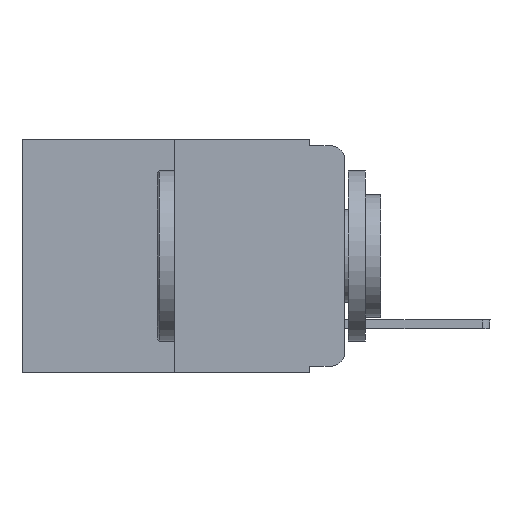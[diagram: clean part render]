
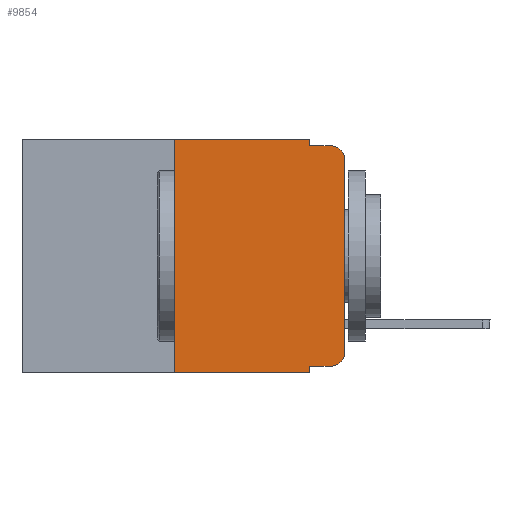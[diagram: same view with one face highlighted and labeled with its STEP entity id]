
A CAD part, left-side view. The second image highlights one B-rep face of the part: STEP entity #9854.
In plain terms, the highlighted planar face has unit normal (-1, 0, 0).
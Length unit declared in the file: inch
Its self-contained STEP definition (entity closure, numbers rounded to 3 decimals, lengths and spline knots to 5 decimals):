
#209 = DIRECTION ( 'NONE',  ( 0., -1., 0. ) ) ;
#552 = VERTEX_POINT ( 'NONE', #6291 ) ;
#686 = VECTOR ( 'NONE', #209, 39.37008 ) ;
#919 = EDGE_CURVE ( 'NONE', #14652, #11674, #9629, .T. ) ;
#1417 = ORIENTED_EDGE ( 'NONE', *, *, #19301, .F. ) ;
#1532 = DIRECTION ( 'NONE',  ( 0., 0., -1. ) ) ;
#1660 = VERTEX_POINT ( 'NONE', #18751 ) ;
#1705 = VERTEX_POINT ( 'NONE', #12756 ) ;
#1905 = EDGE_CURVE ( 'NONE', #5486, #1705, #5115, .T. ) ;
#2225 = EDGE_CURVE ( 'NONE', #14652, #9755, #11635, .T. ) ;
#2271 = ORIENTED_EDGE ( 'NONE', *, *, #5513, .F. ) ;
#2511 = DIRECTION ( 'NONE',  ( -1., 0., 0. ) ) ;
#2537 = CARTESIAN_POINT ( 'NONE',  ( 0., 0.02, -0.01 ) ) ;
#2592 = LINE ( 'NONE', #7316, #13787 ) ;
#2668 = DIRECTION ( 'NONE',  ( -1., 0., 0. ) ) ;
#3148 = EDGE_CURVE ( 'NONE', #552, #21442, #18914, .T. ) ;
#3550 = EDGE_CURVE ( 'NONE', #8674, #1660, #5572, .T. ) ;
#3687 = CARTESIAN_POINT ( 'NONE',  ( 0., 0.051, 0. ) ) ;
#3995 = VECTOR ( 'NONE', #19295, 39.37008 ) ;
#4328 = CARTESIAN_POINT ( 'NONE',  ( 0., 0.25, -0.343 ) ) ;
#5115 = LINE ( 'NONE', #20391, #686 ) ;
#5486 = VERTEX_POINT ( 'NONE', #11490 ) ;
#5513 = EDGE_CURVE ( 'NONE', #10759, #552, #10930, .T. ) ;
#5572 = LINE ( 'NONE', #9108, #3995 ) ;
#5699 = ORIENTED_EDGE ( 'NONE', *, *, #3148, .F. ) ;
#5952 = CARTESIAN_POINT ( 'NONE',  ( 0., 0.051, -0.343 ) ) ;
#6035 = EDGE_CURVE ( 'NONE', #1660, #21442, #16421, .T. ) ;
#6173 = CARTESIAN_POINT ( 'NONE',  ( 0., 0., -0.313 ) ) ;
#6238 = DIRECTION ( 'NONE',  ( 0., 0., -1. ) ) ;
#6291 = CARTESIAN_POINT ( 'NONE',  ( 0., 0.051, -0.01 ) ) ;
#6382 = AXIS2_PLACEMENT_3D ( 'NONE', #12459, #2511, #7522 ) ;
#6492 = CARTESIAN_POINT ( 'NONE',  ( 0., 0.051, 0. ) ) ;
#6511 = VECTOR ( 'NONE', #1532, 39.37008 ) ;
#6634 = ORIENTED_EDGE ( 'NONE', *, *, #18701, .T. ) ;
#7316 = CARTESIAN_POINT ( 'NONE',  ( 0., 0.473, 0. ) ) ;
#7522 = DIRECTION ( 'NONE',  ( 0., 0., -1. ) ) ;
#7699 = CARTESIAN_POINT ( 'NONE',  ( 0., 0.02, -0.03 ) ) ;
#7962 = CARTESIAN_POINT ( 'NONE',  ( 0., 0.25, 0. ) ) ;
#8349 = VECTOR ( 'NONE', #6238, 39.37008 ) ;
#8395 = CIRCLE ( 'NONE', #6382, 0.02 ) ;
#8673 = ORIENTED_EDGE ( 'NONE', *, *, #1905, .T. ) ;
#8674 = VERTEX_POINT ( 'NONE', #6173 ) ;
#9057 = PLANE ( 'NONE',  #16336 ) ;
#9108 = CARTESIAN_POINT ( 'NONE',  ( 0., 0., 0. ) ) ;
#9545 = CARTESIAN_POINT ( 'NONE',  ( 0., 0.051, 0. ) ) ;
#9629 = LINE ( 'NONE', #12203, #13524 ) ;
#9734 = ORIENTED_EDGE ( 'NONE', *, *, #10953, .F. ) ;
#9755 = VERTEX_POINT ( 'NONE', #5952 ) ;
#9854 = ADVANCED_FACE ( 'NONE', ( #20655 ), #9057, .F. ) ;
#9924 = ORIENTED_EDGE ( 'NONE', *, *, #919, .F. ) ;
#10759 = VERTEX_POINT ( 'NONE', #3687 ) ;
#10767 = EDGE_LOOP ( 'NONE', ( #15612, #12100, #5699, #2271, #9734, #9924, #16458, #1417, #8673, #6634 ) ) ;
#10930 = LINE ( 'NONE', #6492, #6511 ) ;
#10953 = EDGE_CURVE ( 'NONE', #11674, #10759, #2592, .T. ) ;
#11490 = CARTESIAN_POINT ( 'NONE',  ( 0., 0.051, -0.333 ) ) ;
#11635 = LINE ( 'NONE', #20192, #20008 ) ;
#11674 = VERTEX_POINT ( 'NONE', #7962 ) ;
#12100 = ORIENTED_EDGE ( 'NONE', *, *, #6035, .T. ) ;
#12203 = CARTESIAN_POINT ( 'NONE',  ( 0., 0.25, 0. ) ) ;
#12459 = CARTESIAN_POINT ( 'NONE',  ( 0., 0.02, -0.313 ) ) ;
#12756 = CARTESIAN_POINT ( 'NONE',  ( 0., 0.02, -0.333 ) ) ;
#12782 = DIRECTION ( 'NONE',  ( 0., 0., -1. ) ) ;
#13524 = VECTOR ( 'NONE', #13876, 39.37008 ) ;
#13584 = LINE ( 'NONE', #9545, #8349 ) ;
#13787 = VECTOR ( 'NONE', #18991, 39.37008 ) ;
#13876 = DIRECTION ( 'NONE',  ( 0., 0., 1. ) ) ;
#13926 = CARTESIAN_POINT ( 'NONE',  ( 0., 0.473, 0. ) ) ;
#14135 = DIRECTION ( 'NONE',  ( 0., 0., -1. ) ) ;
#14652 = VERTEX_POINT ( 'NONE', #4328 ) ;
#15612 = ORIENTED_EDGE ( 'NONE', *, *, #3550, .T. ) ;
#16336 = AXIS2_PLACEMENT_3D ( 'NONE', #13926, #20740, #14135 ) ;
#16421 = CIRCLE ( 'NONE', #19184, 0.02 ) ;
#16458 = ORIENTED_EDGE ( 'NONE', *, *, #2225, .T. ) ;
#16645 = DIRECTION ( 'NONE',  ( 0., -1., 0. ) ) ;
#16929 = DIRECTION ( 'NONE',  ( 0., -1., 0. ) ) ;
#18014 = CARTESIAN_POINT ( 'NONE',  ( 0., 0.051, -0.01 ) ) ;
#18409 = VECTOR ( 'NONE', #16645, 39.37008 ) ;
#18701 = EDGE_CURVE ( 'NONE', #1705, #8674, #8395, .T. ) ;
#18751 = CARTESIAN_POINT ( 'NONE',  ( 0., 0., -0.03 ) ) ;
#18914 = LINE ( 'NONE', #18014, #18409 ) ;
#18991 = DIRECTION ( 'NONE',  ( 0., -1., 0. ) ) ;
#19184 = AXIS2_PLACEMENT_3D ( 'NONE', #7699, #2668, #12782 ) ;
#19295 = DIRECTION ( 'NONE',  ( 0., 0., 1. ) ) ;
#19301 = EDGE_CURVE ( 'NONE', #5486, #9755, #13584, .T. ) ;
#20008 = VECTOR ( 'NONE', #16929, 39.37008 ) ;
#20192 = CARTESIAN_POINT ( 'NONE',  ( 0., 0.473, -0.343 ) ) ;
#20391 = CARTESIAN_POINT ( 'NONE',  ( 0., 0.051, -0.333 ) ) ;
#20655 = FACE_OUTER_BOUND ( 'NONE', #10767, .T. ) ;
#20740 = DIRECTION ( 'NONE',  ( 1., 0., 0. ) ) ;
#21442 = VERTEX_POINT ( 'NONE', #2537 ) ;
